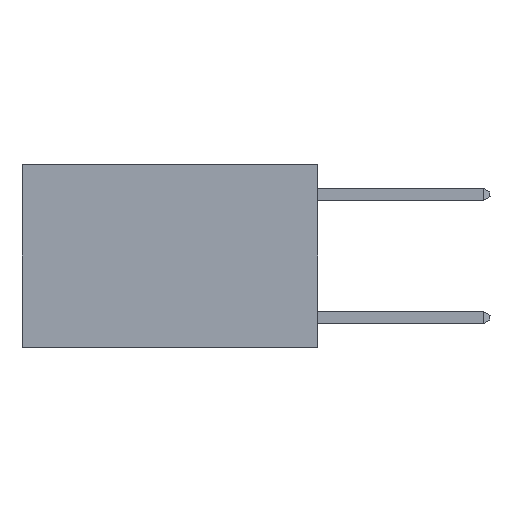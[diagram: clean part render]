
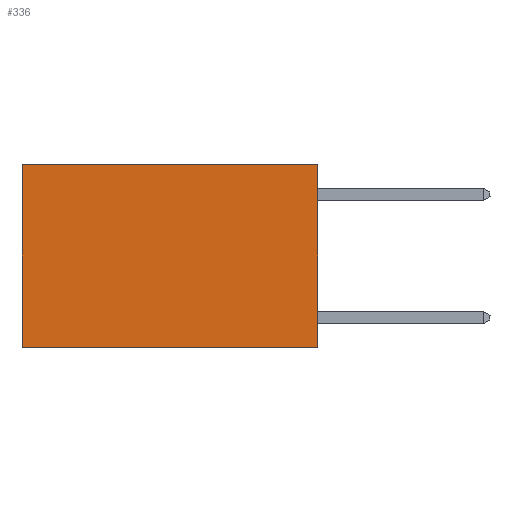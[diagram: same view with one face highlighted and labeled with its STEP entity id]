
A CAD part, left-side view. The second image highlights one B-rep face of the part: STEP entity #336.
In plain terms, the highlighted planar face has unit normal (-1, 0, 0).
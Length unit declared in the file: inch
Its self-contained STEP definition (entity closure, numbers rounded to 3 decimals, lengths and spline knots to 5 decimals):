
#336 = ADVANCED_FACE ( 'NONE', ( #18037 ), #3262, .F. ) ;
#1801 = LINE ( 'NONE', #20298, #6377 ) ;
#3262 = PLANE ( 'NONE',  #14797 ) ;
#3840 = ORIENTED_EDGE ( 'NONE', *, *, #17863, .T. ) ;
#3938 = ORIENTED_EDGE ( 'NONE', *, *, #15625, .F. ) ;
#4660 = CARTESIAN_POINT ( 'NONE',  ( 0.2625, 0., 0. ) ) ;
#4877 = CARTESIAN_POINT ( 'NONE',  ( 0.2625, 0., -0.37 ) ) ;
#5711 = ORIENTED_EDGE ( 'NONE', *, *, #17516, .F. ) ;
#6120 = DIRECTION ( 'NONE',  ( 0., 1., 0. ) ) ;
#6152 = VERTEX_POINT ( 'NONE', #8386 ) ;
#6377 = VECTOR ( 'NONE', #7257, 39.37008 ) ;
#7257 = DIRECTION ( 'NONE',  ( 0., 0., -1. ) ) ;
#8245 = DIRECTION ( 'NONE',  ( 0., 0., -1. ) ) ;
#8386 = CARTESIAN_POINT ( 'NONE',  ( 0.2625, 0.6, -0.37 ) ) ;
#8701 = EDGE_CURVE ( 'NONE', #11157, #6152, #1801, .T. ) ;
#8779 = VECTOR ( 'NONE', #19956, 39.37008 ) ;
#9148 = VECTOR ( 'NONE', #6120, 39.37008 ) ;
#9976 = LINE ( 'NONE', #19645, #21024 ) ;
#11157 = VERTEX_POINT ( 'NONE', #14493 ) ;
#11303 = VERTEX_POINT ( 'NONE', #18509 ) ;
#11315 = DIRECTION ( 'NONE',  ( 1., 0., 0. ) ) ;
#13253 = DIRECTION ( 'NONE',  ( 0., 0., -1. ) ) ;
#14493 = CARTESIAN_POINT ( 'NONE',  ( 0.2625, 0.6, 0. ) ) ;
#14797 = AXIS2_PLACEMENT_3D ( 'NONE', #4660, #11315, #13253 ) ;
#15625 = EDGE_CURVE ( 'NONE', #11303, #18810, #9976, .T. ) ;
#15824 = ORIENTED_EDGE ( 'NONE', *, *, #8701, .T. ) ;
#17516 = EDGE_CURVE ( 'NONE', #18810, #6152, #18310, .T. ) ;
#17863 = EDGE_CURVE ( 'NONE', #11303, #11157, #19821, .T. ) ;
#18037 = FACE_OUTER_BOUND ( 'NONE', #18605, .T. ) ;
#18310 = LINE ( 'NONE', #18739, #8779 ) ;
#18509 = CARTESIAN_POINT ( 'NONE',  ( 0.2625, 0., 0. ) ) ;
#18605 = EDGE_LOOP ( 'NONE', ( #15824, #5711, #3938, #3840 ) ) ;
#18739 = CARTESIAN_POINT ( 'NONE',  ( 0.2625, 0., -0.37 ) ) ;
#18810 = VERTEX_POINT ( 'NONE', #4877 ) ;
#19645 = CARTESIAN_POINT ( 'NONE',  ( 0.2625, 0., 0. ) ) ;
#19821 = LINE ( 'NONE', #21025, #9148 ) ;
#19956 = DIRECTION ( 'NONE',  ( 0., 1., 0. ) ) ;
#20298 = CARTESIAN_POINT ( 'NONE',  ( 0.2625, 0.6, 0. ) ) ;
#21024 = VECTOR ( 'NONE', #8245, 39.37008 ) ;
#21025 = CARTESIAN_POINT ( 'NONE',  ( 0.2625, 0., 0. ) ) ;
